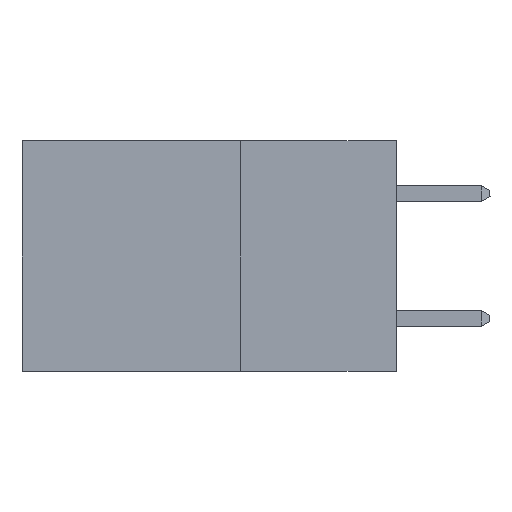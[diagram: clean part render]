
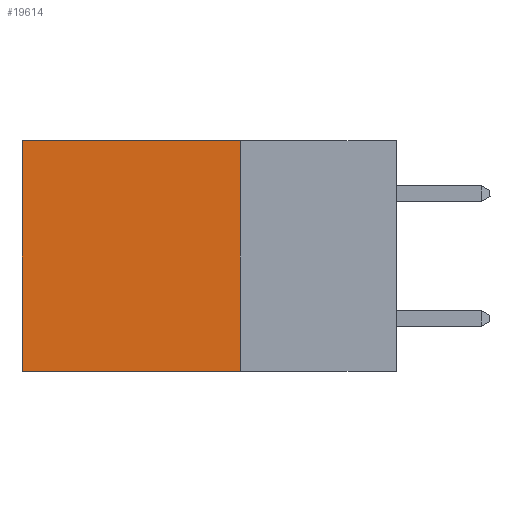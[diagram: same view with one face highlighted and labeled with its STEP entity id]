
A CAD part, left-side view. The second image highlights one B-rep face of the part: STEP entity #19614.
In plain terms, the highlighted planar face has unit normal (-1, 0, 0).
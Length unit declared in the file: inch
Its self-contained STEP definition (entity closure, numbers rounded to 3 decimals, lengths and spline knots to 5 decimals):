
#1744 = CARTESIAN_POINT ( 'NONE',  ( 0.2615, 0.25, -0.37 ) ) ;
#2373 = EDGE_CURVE ( 'NONE', #6447, #20149, #15335, .T. ) ;
#3574 = EDGE_CURVE ( 'NONE', #19163, #8182, #5599, .T. ) ;
#3692 = EDGE_CURVE ( 'NONE', #6447, #19163, #12427, .T. ) ;
#4629 = AXIS2_PLACEMENT_3D ( 'NONE', #8730, #21398, #10539 ) ;
#5599 = LINE ( 'NONE', #1744, #9350 ) ;
#5755 = CARTESIAN_POINT ( 'NONE',  ( 0.2615, 0.25, -0.37 ) ) ;
#6447 = VERTEX_POINT ( 'NONE', #15412 ) ;
#6704 = LINE ( 'NONE', #23024, #21739 ) ;
#6710 = DIRECTION ( 'NONE',  ( 0., 0., -1. ) ) ;
#6884 = PLANE ( 'NONE',  #4629 ) ;
#7047 = VECTOR ( 'NONE', #20316, 39.37008 ) ;
#7725 = ORIENTED_EDGE ( 'NONE', *, *, #2373, .T. ) ;
#8182 = VERTEX_POINT ( 'NONE', #21619 ) ;
#8730 = CARTESIAN_POINT ( 'NONE',  ( 0.2615, 0.25, -0.37 ) ) ;
#9350 = VECTOR ( 'NONE', #16437, 39.37008 ) ;
#10539 = DIRECTION ( 'NONE',  ( 0., 0., -1. ) ) ;
#11030 = CARTESIAN_POINT ( 'NONE',  ( 0.2615, 0.25, -0.37 ) ) ;
#11116 = ORIENTED_EDGE ( 'NONE', *, *, #3574, .F. ) ;
#12427 = LINE ( 'NONE', #5755, #7047 ) ;
#12999 = EDGE_LOOP ( 'NONE', ( #16975, #11116, #21014, #7725 ) ) ;
#15335 = LINE ( 'NONE', #15869, #19573 ) ;
#15412 = CARTESIAN_POINT ( 'NONE',  ( 0.2615, 0.25, 0. ) ) ;
#15869 = CARTESIAN_POINT ( 'NONE',  ( 0.2615, 0.25, 0. ) ) ;
#15889 = DIRECTION ( 'NONE',  ( 0., 1., 0. ) ) ;
#16437 = DIRECTION ( 'NONE',  ( 0., 1., 0. ) ) ;
#16975 = ORIENTED_EDGE ( 'NONE', *, *, #17976, .T. ) ;
#17976 = EDGE_CURVE ( 'NONE', #20149, #8182, #6704, .T. ) ;
#19163 = VERTEX_POINT ( 'NONE', #11030 ) ;
#19464 = FACE_OUTER_BOUND ( 'NONE', #12999, .T. ) ;
#19573 = VECTOR ( 'NONE', #15889, 39.37008 ) ;
#19614 = ADVANCED_FACE ( 'NONE', ( #19464 ), #6884, .F. ) ;
#20149 = VERTEX_POINT ( 'NONE', #20994 ) ;
#20316 = DIRECTION ( 'NONE',  ( 0., 0., -1. ) ) ;
#20994 = CARTESIAN_POINT ( 'NONE',  ( 0.2615, 0.6, 0. ) ) ;
#21014 = ORIENTED_EDGE ( 'NONE', *, *, #3692, .F. ) ;
#21398 = DIRECTION ( 'NONE',  ( 1., 0., 0. ) ) ;
#21619 = CARTESIAN_POINT ( 'NONE',  ( 0.2615, 0.6, -0.37 ) ) ;
#21739 = VECTOR ( 'NONE', #6710, 39.37008 ) ;
#23024 = CARTESIAN_POINT ( 'NONE',  ( 0.2615, 0.6, -0.37 ) ) ;
